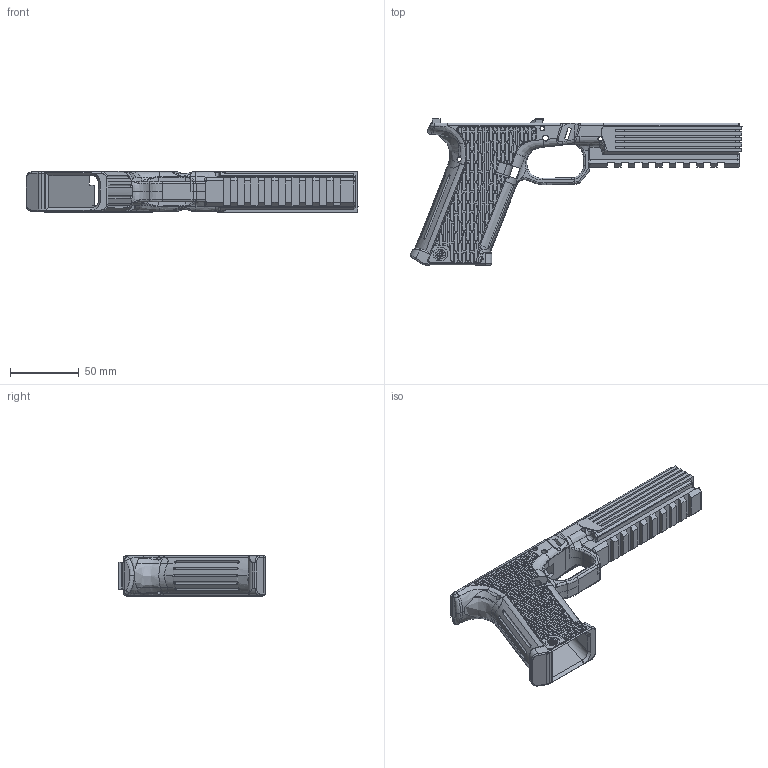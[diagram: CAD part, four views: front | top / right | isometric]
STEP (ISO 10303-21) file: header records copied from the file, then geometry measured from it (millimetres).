
FILE_DESCRIPTION(/* description */ (''),/* implementation_level */ '2;1');
FILE_NAME(/* name */ 'Auto 17L .step',/* time_stamp */ '2021-06-11T08:29:19-06:00',/* author */ (''),/* organization */ (''),/* preprocessor_version */ 'ST-DEVELOPER v18.1',/* originating_system */ 'Autodesk Translation Framework v10.9.0.1377',/* authorisation */ '');
FILE_SCHEMA (('AUTOMOTIVE_DESIGN { 1 0 10303 214 3 1 1 }'));
Products named in the file (1): Auto 17L
Bounding box: 242.07 x 106.5 x 30.34 mm (x, y, z)
Volume: 145438.3 mm3; surface area: 64140.8 mm2
Topology: 1 solids, 3 shells, 3036 faces, 8347 edges, 5415 vertices
Faces by surface type: bspline 1513, plane 1177, cylinder 259, torus 51, sphere 29, cone 7
Full cylindrical faces by diameter (mm): 2 x1, 3 x4, 3.2 x2, 4 x2
Entity records: 121752 total; most frequent: CARTESIAN_POINT 58809, ORIENTED_EDGE 16670, DIRECTION 8955, EDGE_CURVE 8335, VERTEX_POINT 5416, LINE 4405, VECTOR 4405, EDGE_LOOP 3177
